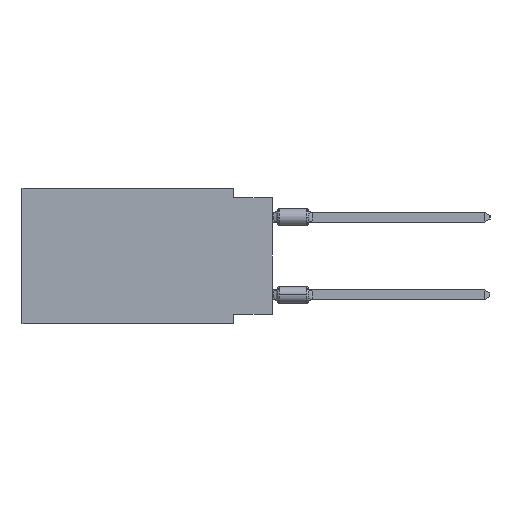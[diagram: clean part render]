
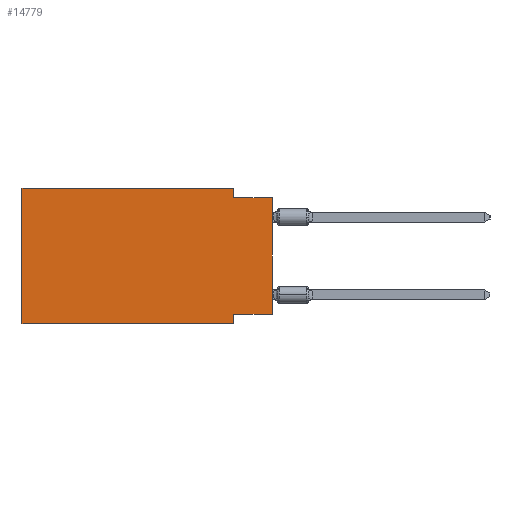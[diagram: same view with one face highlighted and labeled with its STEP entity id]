
A CAD part, left-side view. The second image highlights one B-rep face of the part: STEP entity #14779.
In plain terms, the highlighted planar face has unit normal (-1, 0, 0).
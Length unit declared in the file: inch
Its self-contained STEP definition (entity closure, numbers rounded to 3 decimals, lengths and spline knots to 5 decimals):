
#240 = LINE ( 'NONE', #33669, #57739 ) ;
#1393 = LINE ( 'NONE', #49820, #35413 ) ;
#3974 = VERTEX_POINT ( 'NONE', #19690 ) ;
#4134 = CARTESIAN_POINT ( 'NONE',  ( 0., 0., -0.025 ) ) ;
#5618 = EDGE_CURVE ( 'NONE', #22505, #46558, #14505, .T. ) ;
#6892 = EDGE_CURVE ( 'NONE', #21915, #23040, #25970, .T. ) ;
#7433 = DIRECTION ( 'NONE',  ( 0., 0., -1. ) ) ;
#8081 = PLANE ( 'NONE',  #27808 ) ;
#9688 = VERTEX_POINT ( 'NONE', #31480 ) ;
#9972 = ORIENTED_EDGE ( 'NONE', *, *, #6892, .F. ) ;
#10584 = DIRECTION ( 'NONE',  ( 0., 0., -1. ) ) ;
#12049 = ORIENTED_EDGE ( 'NONE', *, *, #5618, .F. ) ;
#13372 = LINE ( 'NONE', #33484, #53400 ) ;
#14003 = DIRECTION ( 'NONE',  ( 0., 1., 0. ) ) ;
#14154 = VECTOR ( 'NONE', #15906, 39.37008 ) ;
#14505 = LINE ( 'NONE', #4134, #60786 ) ;
#14779 = ADVANCED_FACE ( 'NONE', ( #17173 ), #8081, .F. ) ;
#15906 = DIRECTION ( 'NONE',  ( 0., -1., 0. ) ) ;
#16125 = CARTESIAN_POINT ( 'NONE',  ( 0., 0.1, -0.025 ) ) ;
#17107 = ORIENTED_EDGE ( 'NONE', *, *, #44506, .F. ) ;
#17173 = FACE_OUTER_BOUND ( 'NONE', #55501, .T. ) ;
#17910 = CARTESIAN_POINT ( 'NONE',  ( 0., 0.645, 0. ) ) ;
#19690 = CARTESIAN_POINT ( 'NONE',  ( 0., 0.1, -0.35 ) ) ;
#20308 = VECTOR ( 'NONE', #10584, 39.37008 ) ;
#20979 = CARTESIAN_POINT ( 'NONE',  ( 0., 0.1, -0.35 ) ) ;
#21915 = VERTEX_POINT ( 'NONE', #22496 ) ;
#22496 = CARTESIAN_POINT ( 'NONE',  ( 0., 0.645, 0. ) ) ;
#22505 = VERTEX_POINT ( 'NONE', #16125 ) ;
#22907 = CARTESIAN_POINT ( 'NONE',  ( 0., 0., -0.325 ) ) ;
#23040 = VERTEX_POINT ( 'NONE', #61385 ) ;
#25970 = LINE ( 'NONE', #45800, #14154 ) ;
#26846 = VECTOR ( 'NONE', #58495, 39.37008 ) ;
#27300 = DIRECTION ( 'NONE',  ( 0., 0., 1. ) ) ;
#27808 = AXIS2_PLACEMENT_3D ( 'NONE', #56777, #27879, #7433 ) ;
#27879 = DIRECTION ( 'NONE',  ( 1., 0., 0. ) ) ;
#28615 = LINE ( 'NONE', #38686, #26846 ) ;
#31480 = CARTESIAN_POINT ( 'NONE',  ( 0., 0.645, -0.35 ) ) ;
#33484 = CARTESIAN_POINT ( 'NONE',  ( 0., 0., -0.325 ) ) ;
#33669 = CARTESIAN_POINT ( 'NONE',  ( 0., 0.1, 0. ) ) ;
#34566 = EDGE_CURVE ( 'NONE', #62671, #3974, #55082, .T. ) ;
#34962 = EDGE_CURVE ( 'NONE', #61769, #62671, #13372, .T. ) ;
#35413 = VECTOR ( 'NONE', #50119, 39.37008 ) ;
#35669 = ORIENTED_EDGE ( 'NONE', *, *, #61560, .F. ) ;
#37074 = LINE ( 'NONE', #17910, #40231 ) ;
#38686 = CARTESIAN_POINT ( 'NONE',  ( 0., 0.645, -0.35 ) ) ;
#39185 = DIRECTION ( 'NONE',  ( 0., -1., 0. ) ) ;
#39223 = EDGE_CURVE ( 'NONE', #61769, #46558, #1393, .T. ) ;
#40231 = VECTOR ( 'NONE', #27300, 39.37008 ) ;
#42493 = ORIENTED_EDGE ( 'NONE', *, *, #34962, .F. ) ;
#44403 = DIRECTION ( 'NONE',  ( 0., 0., -1. ) ) ;
#44506 = EDGE_CURVE ( 'NONE', #9688, #21915, #37074, .T. ) ;
#45800 = CARTESIAN_POINT ( 'NONE',  ( 0., 0.645, 0. ) ) ;
#46558 = VERTEX_POINT ( 'NONE', #53062 ) ;
#47016 = CARTESIAN_POINT ( 'NONE',  ( 0., 0.1, -0.325 ) ) ;
#47633 = ORIENTED_EDGE ( 'NONE', *, *, #39223, .T. ) ;
#47768 = EDGE_CURVE ( 'NONE', #9688, #3974, #28615, .T. ) ;
#49820 = CARTESIAN_POINT ( 'NONE',  ( 0., 0., 0. ) ) ;
#50119 = DIRECTION ( 'NONE',  ( 0., 0., 1. ) ) ;
#53062 = CARTESIAN_POINT ( 'NONE',  ( 0., 0., -0.025 ) ) ;
#53400 = VECTOR ( 'NONE', #14003, 39.37008 ) ;
#54116 = ORIENTED_EDGE ( 'NONE', *, *, #34566, .F. ) ;
#55082 = LINE ( 'NONE', #20979, #20308 ) ;
#55501 = EDGE_LOOP ( 'NONE', ( #47633, #12049, #35669, #9972, #17107, #56942, #54116, #42493 ) ) ;
#56777 = CARTESIAN_POINT ( 'NONE',  ( 0., 0.645, 0. ) ) ;
#56942 = ORIENTED_EDGE ( 'NONE', *, *, #47768, .T. ) ;
#57739 = VECTOR ( 'NONE', #44403, 39.37008 ) ;
#58495 = DIRECTION ( 'NONE',  ( 0., -1., 0. ) ) ;
#60786 = VECTOR ( 'NONE', #39185, 39.37008 ) ;
#61385 = CARTESIAN_POINT ( 'NONE',  ( 0., 0.1, 0. ) ) ;
#61560 = EDGE_CURVE ( 'NONE', #23040, #22505, #240, .T. ) ;
#61769 = VERTEX_POINT ( 'NONE', #22907 ) ;
#62671 = VERTEX_POINT ( 'NONE', #47016 ) ;
